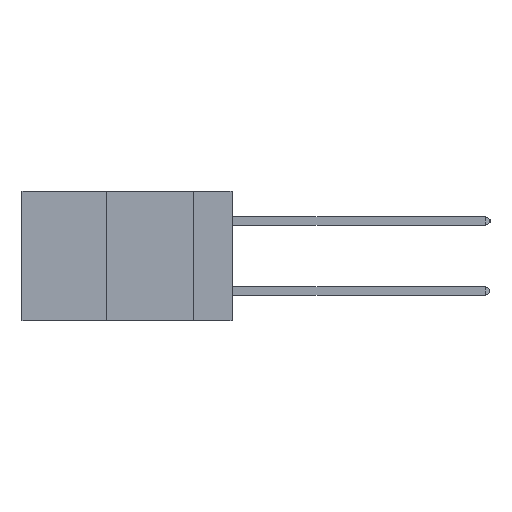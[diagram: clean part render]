
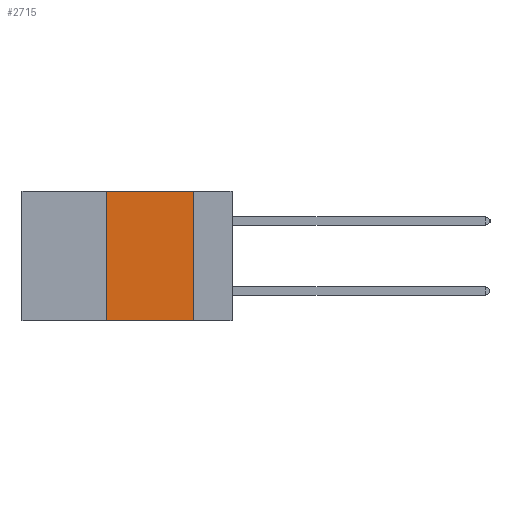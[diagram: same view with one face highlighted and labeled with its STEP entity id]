
A CAD part, left-side view. The second image highlights one B-rep face of the part: STEP entity #2715.
In plain terms, the highlighted planar face has unit normal (-1, 0, 0).
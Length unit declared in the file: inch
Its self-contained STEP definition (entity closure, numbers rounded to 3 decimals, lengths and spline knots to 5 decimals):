
#170 = ORIENTED_EDGE ( 'NONE', *, *, #2578, .F. ) ;
#773 = VERTEX_POINT ( 'NONE', #4248 ) ;
#795 = DIRECTION ( 'NONE',  ( 0., 0., -1. ) ) ;
#946 = VERTEX_POINT ( 'NONE', #8954 ) ;
#1014 = CARTESIAN_POINT ( 'NONE',  ( 0., 0.6, 0. ) ) ;
#1459 = PLANE ( 'NONE',  #5017 ) ;
#1702 = CARTESIAN_POINT ( 'NONE',  ( 0., 0.36, 0. ) ) ;
#1733 = ORIENTED_EDGE ( 'NONE', *, *, #1750, .T. ) ;
#1750 = EDGE_CURVE ( 'NONE', #3104, #946, #9075, .T. ) ;
#1991 = DIRECTION ( 'NONE',  ( 0., -1., 0. ) ) ;
#2578 = EDGE_CURVE ( 'NONE', #3104, #773, #8651, .T. ) ;
#2601 = EDGE_CURVE ( 'NONE', #9598, #946, #7899, .T. ) ;
#2715 = ADVANCED_FACE ( 'NONE', ( #8266 ), #1459, .F. ) ;
#3104 = VERTEX_POINT ( 'NONE', #5936 ) ;
#3209 = VECTOR ( 'NONE', #795, 39.37008 ) ;
#3697 = CARTESIAN_POINT ( 'NONE',  ( 0., 0.11, 0. ) ) ;
#3856 = VECTOR ( 'NONE', #6980, 39.37008 ) ;
#4248 = CARTESIAN_POINT ( 'NONE',  ( 0., 0.36, 0. ) ) ;
#4923 = CARTESIAN_POINT ( 'NONE',  ( 0., 0.11, 0. ) ) ;
#5017 = AXIS2_PLACEMENT_3D ( 'NONE', #11206, #7625, #7906 ) ;
#5806 = DIRECTION ( 'NONE',  ( 0., -1., 0. ) ) ;
#5936 = CARTESIAN_POINT ( 'NONE',  ( 0., 0.36, -0.37 ) ) ;
#6089 = EDGE_LOOP ( 'NONE', ( #7366, #7068, #170, #1733 ) ) ;
#6519 = VECTOR ( 'NONE', #1991, 39.37008 ) ;
#6599 = EDGE_CURVE ( 'NONE', #773, #9598, #6791, .T. ) ;
#6791 = LINE ( 'NONE', #1014, #6519 ) ;
#6980 = DIRECTION ( 'NONE',  ( 0., 0., 1. ) ) ;
#7068 = ORIENTED_EDGE ( 'NONE', *, *, #6599, .F. ) ;
#7366 = ORIENTED_EDGE ( 'NONE', *, *, #2601, .F. ) ;
#7625 = DIRECTION ( 'NONE',  ( 1., 0., 0. ) ) ;
#7899 = LINE ( 'NONE', #4923, #3209 ) ;
#7906 = DIRECTION ( 'NONE',  ( 0., 0., -1. ) ) ;
#8266 = FACE_OUTER_BOUND ( 'NONE', #6089, .T. ) ;
#8651 = LINE ( 'NONE', #1702, #3856 ) ;
#8806 = VECTOR ( 'NONE', #5806, 39.37008 ) ;
#8954 = CARTESIAN_POINT ( 'NONE',  ( 0., 0.11, -0.37 ) ) ;
#9075 = LINE ( 'NONE', #10989, #8806 ) ;
#9598 = VERTEX_POINT ( 'NONE', #3697 ) ;
#10989 = CARTESIAN_POINT ( 'NONE',  ( 0., 0.6, -0.37 ) ) ;
#11206 = CARTESIAN_POINT ( 'NONE',  ( 0., 0.6, 0. ) ) ;
